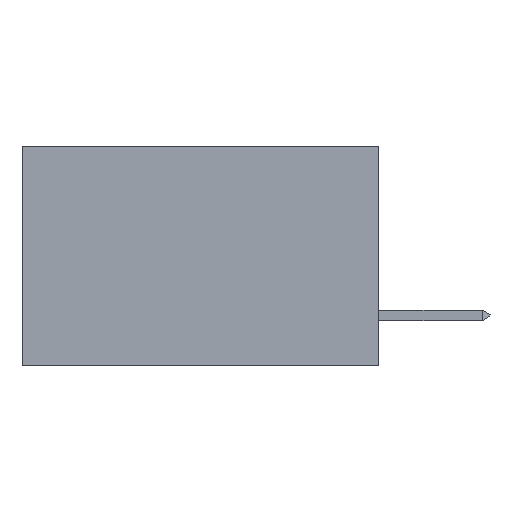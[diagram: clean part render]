
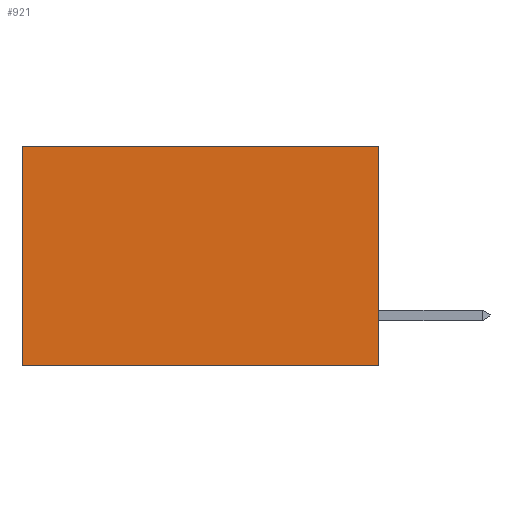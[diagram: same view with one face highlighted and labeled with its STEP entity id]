
A CAD part, left-side view. The second image highlights one B-rep face of the part: STEP entity #921.
In plain terms, the highlighted planar face has unit normal (-1, 0, 0).
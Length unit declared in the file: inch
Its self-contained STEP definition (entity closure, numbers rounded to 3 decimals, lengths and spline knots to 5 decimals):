
#9 = VECTOR ( 'NONE', #5856, 39.37008 ) ;
#55 = DIRECTION ( 'NONE',  ( 0., 0., -1. ) ) ;
#370 = CARTESIAN_POINT ( 'NONE',  ( 0.2615, 0., -0.37 ) ) ;
#807 = CARTESIAN_POINT ( 'NONE',  ( 0.2615, 0., 0. ) ) ;
#921 = ADVANCED_FACE ( 'NONE', ( #4632 ), #10217, .F. ) ;
#1681 = VERTEX_POINT ( 'NONE', #9096 ) ;
#1972 = ORIENTED_EDGE ( 'NONE', *, *, #6307, .T. ) ;
#2342 = EDGE_CURVE ( 'NONE', #8219, #5209, #2493, .T. ) ;
#2394 = CARTESIAN_POINT ( 'NONE',  ( 0.2615, 0.6, -0.37 ) ) ;
#2493 = LINE ( 'NONE', #2394, #9631 ) ;
#2568 = LINE ( 'NONE', #5804, #9 ) ;
#3004 = EDGE_CURVE ( 'NONE', #1681, #5209, #3056, .T. ) ;
#3032 = CARTESIAN_POINT ( 'NONE',  ( 0.2615, 0.6, -0.37 ) ) ;
#3056 = LINE ( 'NONE', #7799, #8974 ) ;
#3569 = CARTESIAN_POINT ( 'NONE',  ( 0.2615, 0., 0. ) ) ;
#4556 = ORIENTED_EDGE ( 'NONE', *, *, #3004, .F. ) ;
#4632 = FACE_OUTER_BOUND ( 'NONE', #5391, .T. ) ;
#4763 = ORIENTED_EDGE ( 'NONE', *, *, #2342, .T. ) ;
#5041 = EDGE_CURVE ( 'NONE', #6951, #1681, #2568, .T. ) ;
#5209 = VERTEX_POINT ( 'NONE', #3032 ) ;
#5214 = AXIS2_PLACEMENT_3D ( 'NONE', #370, #7757, #7705 ) ;
#5391 = EDGE_LOOP ( 'NONE', ( #4763, #4556, #9745, #1972 ) ) ;
#5804 = CARTESIAN_POINT ( 'NONE',  ( 0.2615, 0., -0.37 ) ) ;
#5856 = DIRECTION ( 'NONE',  ( 0., 0., -1. ) ) ;
#6307 = EDGE_CURVE ( 'NONE', #6951, #8219, #7669, .T. ) ;
#6951 = VERTEX_POINT ( 'NONE', #807 ) ;
#7669 = LINE ( 'NONE', #3569, #8883 ) ;
#7705 = DIRECTION ( 'NONE',  ( 0., 0., -1. ) ) ;
#7757 = DIRECTION ( 'NONE',  ( 1., 0., 0. ) ) ;
#7799 = CARTESIAN_POINT ( 'NONE',  ( 0.2615, 0., -0.37 ) ) ;
#8219 = VERTEX_POINT ( 'NONE', #9240 ) ;
#8883 = VECTOR ( 'NONE', #9332, 39.37008 ) ;
#8974 = VECTOR ( 'NONE', #10256, 39.37008 ) ;
#9096 = CARTESIAN_POINT ( 'NONE',  ( 0.2615, 0., -0.37 ) ) ;
#9240 = CARTESIAN_POINT ( 'NONE',  ( 0.2615, 0.6, 0. ) ) ;
#9332 = DIRECTION ( 'NONE',  ( 0., 1., 0. ) ) ;
#9631 = VECTOR ( 'NONE', #55, 39.37008 ) ;
#9745 = ORIENTED_EDGE ( 'NONE', *, *, #5041, .F. ) ;
#10217 = PLANE ( 'NONE',  #5214 ) ;
#10256 = DIRECTION ( 'NONE',  ( 0., 1., 0. ) ) ;
